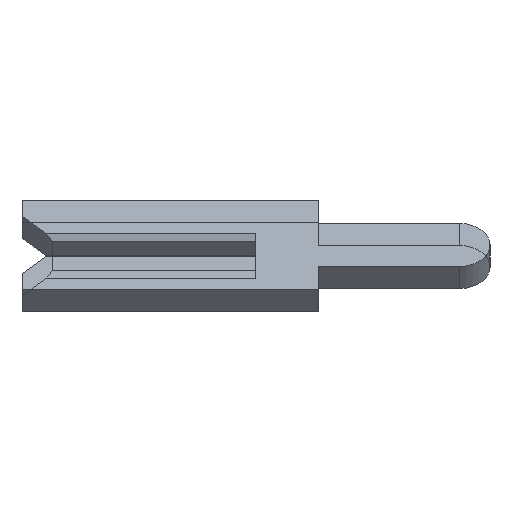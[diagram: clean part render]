
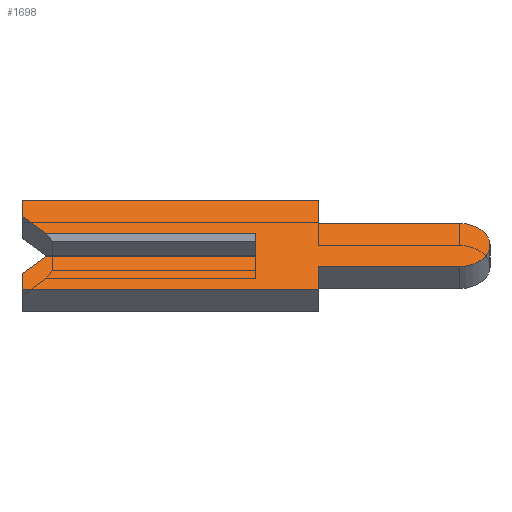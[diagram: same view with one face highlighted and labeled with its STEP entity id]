
A CAD part, left-side view. The second image highlights one B-rep face of the part: STEP entity #1698.
In plain terms, the highlighted face is planar.
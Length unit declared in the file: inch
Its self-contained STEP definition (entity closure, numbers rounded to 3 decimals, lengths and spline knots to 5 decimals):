
#13 = LINE ( 'NONE', #3609, #4030 ) ;
#40 = CARTESIAN_POINT ( 'NONE',  ( -0.01, -0.04, -0.04 ) ) ;
#95 = CARTESIAN_POINT ( 'NONE',  ( -0.01, -0.1305, 0. ) ) ;
#167 = VERTEX_POINT ( 'NONE', #245 ) ;
#176 = EDGE_CURVE ( 'NONE', #2901, #2349, #2238, .T. ) ;
#198 = DIRECTION ( 'NONE',  ( 0., 0., 1. ) ) ;
#239 = EDGE_CURVE ( 'NONE', #1863, #167, #4320, .T. ) ;
#245 = CARTESIAN_POINT ( 'NONE',  ( -0.01, 0., 0.01 ) ) ;
#341 = EDGE_CURVE ( 'NONE', #2565, #2901, #750, .T. ) ;
#383 = CARTESIAN_POINT ( 'NONE',  ( -0.01, -0.04, 0.04 ) ) ;
#415 = DIRECTION ( 'NONE',  ( 0., 1., 0. ) ) ;
#417 = VECTOR ( 'NONE', #552, 39.37008 ) ;
#454 = DIRECTION ( 'NONE',  ( 1., 0., 0. ) ) ;
#502 = EDGE_CURVE ( 'NONE', #1127, #167, #2689, .T. ) ;
#514 = ORIENTED_EDGE ( 'NONE', *, *, #3737, .F. ) ;
#537 = CARTESIAN_POINT ( 'NONE',  ( -0.01, 0.1305, -0.0065 ) ) ;
#552 = DIRECTION ( 'NONE',  ( 0., -1., 0. ) ) ;
#559 = DIRECTION ( 'NONE',  ( 0., 0., 1. ) ) ;
#564 = VERTEX_POINT ( 'NONE', #3178 ) ;
#571 = CARTESIAN_POINT ( 'NONE',  ( -0.01, 0.15, 0.04 ) ) ;
#572 = ORIENTED_EDGE ( 'NONE', *, *, #2627, .F. ) ;
#682 = DIRECTION ( 'NONE',  ( 0., -1., 0. ) ) ;
#726 = CARTESIAN_POINT ( 'NONE',  ( -0.01, -0.1305, 0. ) ) ;
#750 = LINE ( 'NONE', #3795, #815 ) ;
#815 = VECTOR ( 'NONE', #559, 39.37008 ) ;
#864 = CARTESIAN_POINT ( 'NONE',  ( -0.01, 0.15, -0.026 ) ) ;
#968 = DIRECTION ( 'NONE',  ( 0., 0.707, 0.707 ) ) ;
#1020 = CARTESIAN_POINT ( 'NONE',  ( -0.01, -0.1305, -0.01 ) ) ;
#1030 = VECTOR ( 'NONE', #2174, 39.37008 ) ;
#1057 = DIRECTION ( 'NONE',  ( 0., 0., -1. ) ) ;
#1069 = EDGE_CURVE ( 'NONE', #564, #1863, #2638, .T. ) ;
#1086 = DIRECTION ( 'NONE',  ( 1., 0., 0. ) ) ;
#1088 = LINE ( 'NONE', #2210, #1711 ) ;
#1127 = VERTEX_POINT ( 'NONE', #3886 ) ;
#1133 = CARTESIAN_POINT ( 'NONE',  ( -0.01, -0.04, 0.04 ) ) ;
#1170 = CARTESIAN_POINT ( 'NONE',  ( -0.01, 0.15, -0.04 ) ) ;
#1201 = VECTOR ( 'NONE', #2456, 39.37008 ) ;
#1235 = CARTESIAN_POINT ( 'NONE',  ( -0.01, -0.04, -0.04 ) ) ;
#1370 = ORIENTED_EDGE ( 'NONE', *, *, #502, .T. ) ;
#1409 = EDGE_CURVE ( 'NONE', #4506, #2919, #4202, .T. ) ;
#1472 = ORIENTED_EDGE ( 'NONE', *, *, #4462, .F. ) ;
#1527 = CARTESIAN_POINT ( 'NONE',  ( -0.01, 0.15, 0.026 ) ) ;
#1557 = VERTEX_POINT ( 'NONE', #2560 ) ;
#1560 = EDGE_CURVE ( 'NONE', #2349, #1557, #1824, .T. ) ;
#1605 = ORIENTED_EDGE ( 'NONE', *, *, #1887, .F. ) ;
#1660 = CARTESIAN_POINT ( 'NONE',  ( -0.01, -0.04, -0.0195 ) ) ;
#1668 = VECTOR ( 'NONE', #682, 39.37008 ) ;
#1698 = ADVANCED_FACE ( 'NONE', ( #2741 ), #3594, .F. ) ;
#1711 = VECTOR ( 'NONE', #415, 39.37008 ) ;
#1739 = AXIS2_PLACEMENT_3D ( 'NONE', #95, #454, #3732 ) ;
#1824 = LINE ( 'NONE', #383, #1030 ) ;
#1863 = VERTEX_POINT ( 'NONE', #3947 ) ;
#1881 = DIRECTION ( 'NONE',  ( 0., 0., 1. ) ) ;
#1883 = LINE ( 'NONE', #537, #4371 ) ;
#1887 = EDGE_CURVE ( 'NONE', #2919, #2337, #1088, .T. ) ;
#1934 = EDGE_LOOP ( 'NONE', ( #1370, #4189, #1973, #514, #4274, #1605, #2158, #3101, #572, #4144, #4016, #4388, #3056, #1472 ) ) ;
#1973 = ORIENTED_EDGE ( 'NONE', *, *, #1069, .F. ) ;
#1985 = EDGE_CURVE ( 'NONE', #2337, #3009, #13, .T. ) ;
#2082 = VERTEX_POINT ( 'NONE', #4429 ) ;
#2158 = ORIENTED_EDGE ( 'NONE', *, *, #1409, .F. ) ;
#2174 = DIRECTION ( 'NONE',  ( 0., 0., -1. ) ) ;
#2176 = VECTOR ( 'NONE', #1057, 39.37008 ) ;
#2210 = CARTESIAN_POINT ( 'NONE',  ( -0.01, 0.15, -0.04 ) ) ;
#2223 = EDGE_CURVE ( 'NONE', #2780, #4506, #3476, .T. ) ;
#2238 = LINE ( 'NONE', #571, #4541 ) ;
#2301 = VECTOR ( 'NONE', #198, 39.37008 ) ;
#2337 = VERTEX_POINT ( 'NONE', #1170 ) ;
#2349 = VERTEX_POINT ( 'NONE', #1133 ) ;
#2456 = DIRECTION ( 'NONE',  ( 0., 1., 0. ) ) ;
#2560 = CARTESIAN_POINT ( 'NONE',  ( -0.01, -0.04, 0.0195 ) ) ;
#2565 = VERTEX_POINT ( 'NONE', #1527 ) ;
#2627 = EDGE_CURVE ( 'NONE', #2082, #2780, #3804, .T. ) ;
#2638 = LINE ( 'NONE', #1020, #3640 ) ;
#2689 = LINE ( 'NONE', #3562, #1668 ) ;
#2741 = FACE_OUTER_BOUND ( 'NONE', #1934, .T. ) ;
#2780 = VERTEX_POINT ( 'NONE', #3380 ) ;
#2853 = DIRECTION ( 'NONE',  ( 0., -1., 0. ) ) ;
#2900 = AXIS2_PLACEMENT_3D ( 'NONE', #726, #1086, #2902 ) ;
#2901 = VERTEX_POINT ( 'NONE', #4150 ) ;
#2902 = DIRECTION ( 'NONE',  ( 0., 0., -1. ) ) ;
#2919 = VERTEX_POINT ( 'NONE', #1235 ) ;
#3009 = VERTEX_POINT ( 'NONE', #864 ) ;
#3056 = ORIENTED_EDGE ( 'NONE', *, *, #341, .F. ) ;
#3082 = VECTOR ( 'NONE', #968, 39.37008 ) ;
#3091 = DIRECTION ( 'NONE',  ( 0., -0.707, 0.707 ) ) ;
#3101 = ORIENTED_EDGE ( 'NONE', *, *, #2223, .F. ) ;
#3178 = CARTESIAN_POINT ( 'NONE',  ( -0.01, 0.134, -0.01 ) ) ;
#3380 = CARTESIAN_POINT ( 'NONE',  ( -0.01, -0.1305, -0.0195 ) ) ;
#3438 = EDGE_CURVE ( 'NONE', #1557, #2082, #4022, .T. ) ;
#3447 = DIRECTION ( 'NONE',  ( 0., -1., 0. ) ) ;
#3476 = LINE ( 'NONE', #4259, #1201 ) ;
#3562 = CARTESIAN_POINT ( 'NONE',  ( -0.01, 0.15, 0.01 ) ) ;
#3594 = PLANE ( 'NONE',  #2900 ) ;
#3609 = CARTESIAN_POINT ( 'NONE',  ( -0.01, 0.15, -0.026 ) ) ;
#3640 = VECTOR ( 'NONE', #2853, 39.37008 ) ;
#3732 = DIRECTION ( 'NONE',  ( 0., 0., -1. ) ) ;
#3737 = EDGE_CURVE ( 'NONE', #3009, #564, #1883, .T. ) ;
#3795 = CARTESIAN_POINT ( 'NONE',  ( -0.01, 0.15, 0.026 ) ) ;
#3804 = CIRCLE ( 'NONE', #1739, 0.0195 ) ;
#3886 = CARTESIAN_POINT ( 'NONE',  ( -0.01, 0.134, 0.01 ) ) ;
#3947 = CARTESIAN_POINT ( 'NONE',  ( -0.01, 0., -0.01 ) ) ;
#4016 = ORIENTED_EDGE ( 'NONE', *, *, #1560, .F. ) ;
#4022 = LINE ( 'NONE', #4498, #417 ) ;
#4030 = VECTOR ( 'NONE', #1881, 39.37008 ) ;
#4144 = ORIENTED_EDGE ( 'NONE', *, *, #3438, .F. ) ;
#4150 = CARTESIAN_POINT ( 'NONE',  ( -0.01, 0.15, 0.04 ) ) ;
#4174 = CARTESIAN_POINT ( 'NONE',  ( -0.01, 0., 0.0065 ) ) ;
#4184 = CARTESIAN_POINT ( 'NONE',  ( -0.01, 0.1305, 0.0065 ) ) ;
#4189 = ORIENTED_EDGE ( 'NONE', *, *, #239, .F. ) ;
#4195 = LINE ( 'NONE', #4184, #3082 ) ;
#4202 = LINE ( 'NONE', #40, #2176 ) ;
#4259 = CARTESIAN_POINT ( 'NONE',  ( -0.01, -0.04, -0.0195 ) ) ;
#4274 = ORIENTED_EDGE ( 'NONE', *, *, #1985, .F. ) ;
#4320 = LINE ( 'NONE', #4174, #2301 ) ;
#4371 = VECTOR ( 'NONE', #3091, 39.37008 ) ;
#4388 = ORIENTED_EDGE ( 'NONE', *, *, #176, .F. ) ;
#4429 = CARTESIAN_POINT ( 'NONE',  ( -0.01, -0.1305, 0.0195 ) ) ;
#4462 = EDGE_CURVE ( 'NONE', #1127, #2565, #4195, .T. ) ;
#4498 = CARTESIAN_POINT ( 'NONE',  ( -0.01, -0.04, 0.0195 ) ) ;
#4506 = VERTEX_POINT ( 'NONE', #1660 ) ;
#4541 = VECTOR ( 'NONE', #3447, 39.37008 ) ;
